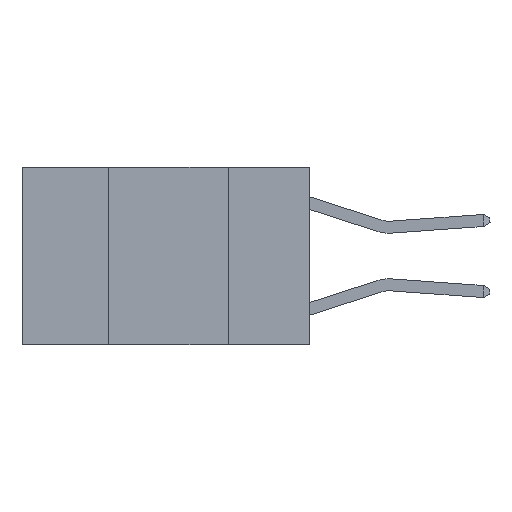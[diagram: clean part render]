
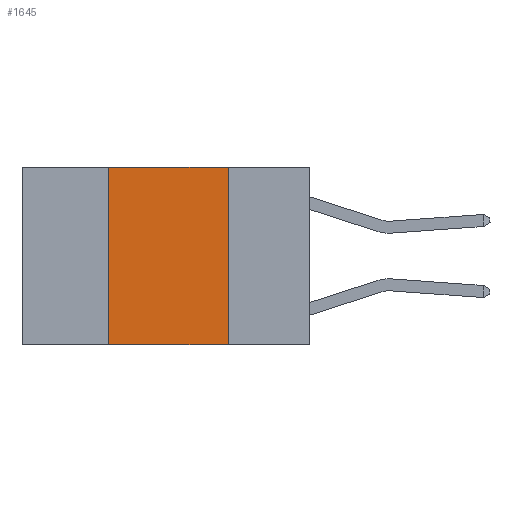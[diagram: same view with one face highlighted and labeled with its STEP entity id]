
A CAD part, left-side view. The second image highlights one B-rep face of the part: STEP entity #1645.
In plain terms, the highlighted planar face has unit normal (-1, 0, 0).
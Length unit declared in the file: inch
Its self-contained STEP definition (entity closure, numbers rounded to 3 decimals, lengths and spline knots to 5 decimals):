
#89 = LINE ( 'NONE', #3642, #2227 ) ;
#98 = LINE ( 'NONE', #555, #4538 ) ;
#356 = LINE ( 'NONE', #4900, #2519 ) ;
#555 = CARTESIAN_POINT ( 'NONE',  ( 0., 0.6, 0. ) ) ;
#556 = EDGE_CURVE ( 'NONE', #1320, #1107, #98, .T. ) ;
#711 = ORIENTED_EDGE ( 'NONE', *, *, #874, .T. ) ;
#858 = EDGE_CURVE ( 'NONE', #1107, #1129, #2786, .T. ) ;
#870 = EDGE_CURVE ( 'NONE', #5097, #1320, #356, .T. ) ;
#874 = EDGE_CURVE ( 'NONE', #5097, #1129, #89, .T. ) ;
#1107 = VERTEX_POINT ( 'NONE', #7864 ) ;
#1129 = VERTEX_POINT ( 'NONE', #8435 ) ;
#1159 = DIRECTION ( 'NONE',  ( 0., 0., -1. ) ) ;
#1320 = VERTEX_POINT ( 'NONE', #3197 ) ;
#1645 = ADVANCED_FACE ( 'NONE', ( #8221 ), #6646, .F. ) ;
#2176 = ORIENTED_EDGE ( 'NONE', *, *, #556, .F. ) ;
#2191 = ORIENTED_EDGE ( 'NONE', *, *, #870, .F. ) ;
#2227 = VECTOR ( 'NONE', #4484, 39.37008 ) ;
#2357 = ORIENTED_EDGE ( 'NONE', *, *, #858, .F. ) ;
#2519 = VECTOR ( 'NONE', #6993, 39.37008 ) ;
#2786 = LINE ( 'NONE', #8699, #4735 ) ;
#3197 = CARTESIAN_POINT ( 'NONE',  ( 0., 0.42, 0. ) ) ;
#3642 = CARTESIAN_POINT ( 'NONE',  ( 0., 0.6, -0.37 ) ) ;
#4484 = DIRECTION ( 'NONE',  ( 0., -1., 0. ) ) ;
#4538 = VECTOR ( 'NONE', #7763, 39.37008 ) ;
#4679 = CARTESIAN_POINT ( 'NONE',  ( 0., 0.42, -0.37 ) ) ;
#4735 = VECTOR ( 'NONE', #1159, 39.37008 ) ;
#4900 = CARTESIAN_POINT ( 'NONE',  ( 0., 0.42, 0. ) ) ;
#5097 = VERTEX_POINT ( 'NONE', #4679 ) ;
#5312 = AXIS2_PLACEMENT_3D ( 'NONE', #8977, #6637, #6556 ) ;
#6556 = DIRECTION ( 'NONE',  ( 0., 0., -1. ) ) ;
#6637 = DIRECTION ( 'NONE',  ( 1., 0., 0. ) ) ;
#6646 = PLANE ( 'NONE',  #5312 ) ;
#6993 = DIRECTION ( 'NONE',  ( 0., 0., 1. ) ) ;
#7763 = DIRECTION ( 'NONE',  ( 0., -1., 0. ) ) ;
#7834 = EDGE_LOOP ( 'NONE', ( #2357, #2176, #2191, #711 ) ) ;
#7864 = CARTESIAN_POINT ( 'NONE',  ( 0., 0.17, 0. ) ) ;
#8221 = FACE_OUTER_BOUND ( 'NONE', #7834, .T. ) ;
#8435 = CARTESIAN_POINT ( 'NONE',  ( 0., 0.17, -0.37 ) ) ;
#8699 = CARTESIAN_POINT ( 'NONE',  ( 0., 0.17, 0. ) ) ;
#8977 = CARTESIAN_POINT ( 'NONE',  ( 0., 0.6, 0. ) ) ;
